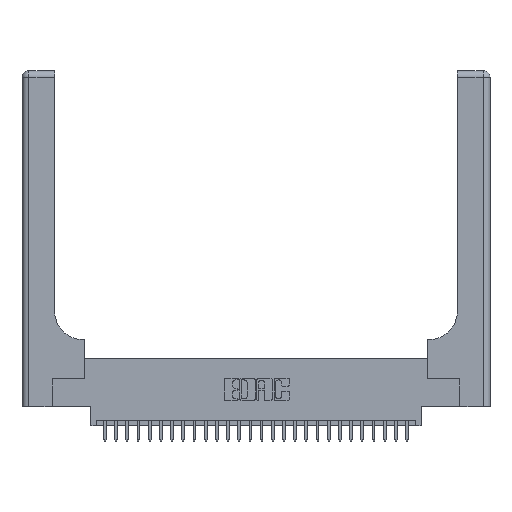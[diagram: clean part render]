
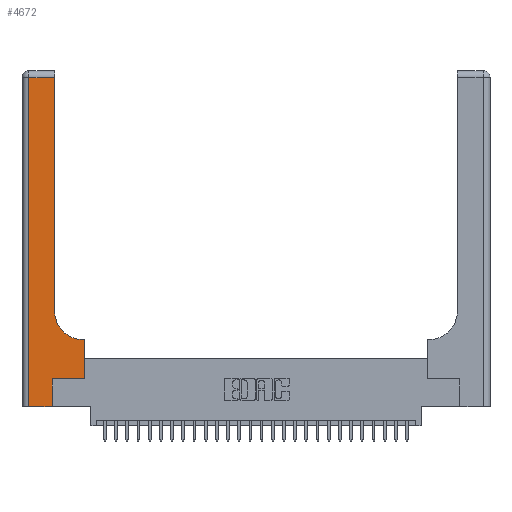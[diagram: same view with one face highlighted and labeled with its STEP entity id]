
A CAD part, top view. The second image highlights one B-rep face of the part: STEP entity #4672.
In plain terms, the highlighted planar face has unit normal (0, 0, 1).
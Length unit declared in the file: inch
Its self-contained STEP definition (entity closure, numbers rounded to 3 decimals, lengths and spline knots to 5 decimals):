
#193 = EDGE_CURVE ( 'NONE', #7510, #13643, #15916, .T. ) ;
#650 = ORIENTED_EDGE ( 'NONE', *, *, #6994, .T. ) ;
#657 = CARTESIAN_POINT ( 'NONE',  ( 0., 3., 0.37 ) ) ;
#881 = DIRECTION ( 'NONE',  ( 0., 1., 0. ) ) ;
#1402 = VECTOR ( 'NONE', #17085, 39.37008 ) ;
#1457 = DIRECTION ( 'NONE',  ( 0., -1., 0. ) ) ;
#1685 = CARTESIAN_POINT ( 'NONE',  ( 0.06, 0., 0.37 ) ) ;
#1768 = DIRECTION ( 'NONE',  ( 1., 0., 0. ) ) ;
#1876 = VECTOR ( 'NONE', #19272, 39.37008 ) ;
#2780 = LINE ( 'NONE', #8583, #7370 ) ;
#3013 = EDGE_CURVE ( 'NONE', #15797, #9282, #26049, .T. ) ;
#3059 = FACE_OUTER_BOUND ( 'NONE', #15293, .T. ) ;
#3144 = EDGE_CURVE ( 'NONE', #24354, #15797, #14047, .T. ) ;
#3611 = VECTOR ( 'NONE', #1457, 39.37008 ) ;
#3672 = CARTESIAN_POINT ( 'NONE',  ( 0.2915, 2.94, 0.37 ) ) ;
#4561 = VECTOR ( 'NONE', #21517, 39.37008 ) ;
#4672 = ADVANCED_FACE ( 'NONE', ( #3059 ), #25319, .F. ) ;
#4695 = VERTEX_POINT ( 'NONE', #4844 ) ;
#4762 = VECTOR ( 'NONE', #15380, 39.37008 ) ;
#4799 = CARTESIAN_POINT ( 'NONE',  ( 0., 2.94, 0.37 ) ) ;
#4844 = CARTESIAN_POINT ( 'NONE',  ( 0.2915, 0.85, 0.37 ) ) ;
#5880 = CARTESIAN_POINT ( 'NONE',  ( 0.269, 0., 0.37 ) ) ;
#6994 = EDGE_CURVE ( 'NONE', #13643, #24354, #13776, .T. ) ;
#7370 = VECTOR ( 'NONE', #1768, 39.37008 ) ;
#7510 = VERTEX_POINT ( 'NONE', #3672 ) ;
#8583 = CARTESIAN_POINT ( 'NONE',  ( 0.269, 0.25, 0.37 ) ) ;
#8662 = EDGE_CURVE ( 'NONE', #9282, #27222, #2780, .T. ) ;
#9282 = VERTEX_POINT ( 'NONE', #10503 ) ;
#10006 = DIRECTION ( 'NONE',  ( 1., 0., 0. ) ) ;
#10257 = VERTEX_POINT ( 'NONE', #23700 ) ;
#10503 = CARTESIAN_POINT ( 'NONE',  ( 0.269, 0.25, 0.37 ) ) ;
#10956 = VERTEX_POINT ( 'NONE', #17338 ) ;
#12956 = VECTOR ( 'NONE', #881, 39.37008 ) ;
#13261 = CARTESIAN_POINT ( 'NONE',  ( 0.5585, 0.25, 0.37 ) ) ;
#13643 = VERTEX_POINT ( 'NONE', #27712 ) ;
#13776 = LINE ( 'NONE', #28432, #3611 ) ;
#14047 = LINE ( 'NONE', #25176, #4561 ) ;
#14144 = EDGE_CURVE ( 'NONE', #27222, #10956, #14858, .T. ) ;
#14185 = ORIENTED_EDGE ( 'NONE', *, *, #3013, .T. ) ;
#14765 = DIRECTION ( 'NONE',  ( 0., 0., -1. ) ) ;
#14858 = LINE ( 'NONE', #23634, #1876 ) ;
#15293 = EDGE_LOOP ( 'NONE', ( #18800, #23616, #650, #22142, #14185, #26158, #16460, #17038, #22358 ) ) ;
#15380 = DIRECTION ( 'NONE',  ( -1., 0., 0. ) ) ;
#15506 = CARTESIAN_POINT ( 'NONE',  ( 0.269, 0., 0.37 ) ) ;
#15572 = AXIS2_PLACEMENT_3D ( 'NONE', #25891, #14765, #10006 ) ;
#15797 = VERTEX_POINT ( 'NONE', #15506 ) ;
#15916 = LINE ( 'NONE', #4799, #21935 ) ;
#16460 = ORIENTED_EDGE ( 'NONE', *, *, #14144, .T. ) ;
#17038 = ORIENTED_EDGE ( 'NONE', *, *, #25512, .T. ) ;
#17085 = DIRECTION ( 'NONE',  ( 0., 1., 0. ) ) ;
#17338 = CARTESIAN_POINT ( 'NONE',  ( 0.5585, 0.6, 0.37 ) ) ;
#18800 = ORIENTED_EDGE ( 'NONE', *, *, #24226, .T. ) ;
#19272 = DIRECTION ( 'NONE',  ( 0., 1., 0. ) ) ;
#20509 = DIRECTION ( 'NONE',  ( -1., 0., 0. ) ) ;
#21517 = DIRECTION ( 'NONE',  ( 1., 0., 0. ) ) ;
#21935 = VECTOR ( 'NONE', #20509, 39.37008 ) ;
#22142 = ORIENTED_EDGE ( 'NONE', *, *, #3144, .T. ) ;
#22358 = ORIENTED_EDGE ( 'NONE', *, *, #28184, .T. ) ;
#23225 = DIRECTION ( 'NONE',  ( -1., 0., 0. ) ) ;
#23326 = CARTESIAN_POINT ( 'NONE',  ( 0.2915, 3., 0.37 ) ) ;
#23515 = LINE ( 'NONE', #23326, #12956 ) ;
#23616 = ORIENTED_EDGE ( 'NONE', *, *, #193, .T. ) ;
#23634 = CARTESIAN_POINT ( 'NONE',  ( 0.5585, 0.25, 0.37 ) ) ;
#23670 = AXIS2_PLACEMENT_3D ( 'NONE', #657, #25767, #23225 ) ;
#23700 = CARTESIAN_POINT ( 'NONE',  ( 0.5415, 0.6, 0.37 ) ) ;
#24226 = EDGE_CURVE ( 'NONE', #4695, #7510, #23515, .T. ) ;
#24354 = VERTEX_POINT ( 'NONE', #1685 ) ;
#25176 = CARTESIAN_POINT ( 'NONE',  ( 0., 0., 0.37 ) ) ;
#25319 = PLANE ( 'NONE',  #23670 ) ;
#25512 = EDGE_CURVE ( 'NONE', #10956, #10257, #28755, .T. ) ;
#25767 = DIRECTION ( 'NONE',  ( 0., 0., -1. ) ) ;
#25891 = CARTESIAN_POINT ( 'NONE',  ( 0.5415, 0.85, 0.37 ) ) ;
#26049 = LINE ( 'NONE', #5880, #1402 ) ;
#26114 = CARTESIAN_POINT ( 'NONE',  ( 0.2915, 0.6, 0.37 ) ) ;
#26158 = ORIENTED_EDGE ( 'NONE', *, *, #8662, .T. ) ;
#26863 = CIRCLE ( 'NONE', #15572, 0.25 ) ;
#27222 = VERTEX_POINT ( 'NONE', #13261 ) ;
#27712 = CARTESIAN_POINT ( 'NONE',  ( 0.06, 2.94, 0.37 ) ) ;
#28184 = EDGE_CURVE ( 'NONE', #10257, #4695, #26863, .T. ) ;
#28432 = CARTESIAN_POINT ( 'NONE',  ( 0.06, 3., 0.37 ) ) ;
#28755 = LINE ( 'NONE', #26114, #4762 ) ;
